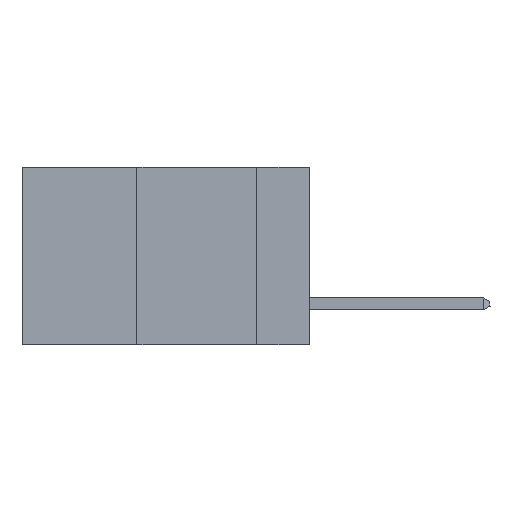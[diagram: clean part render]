
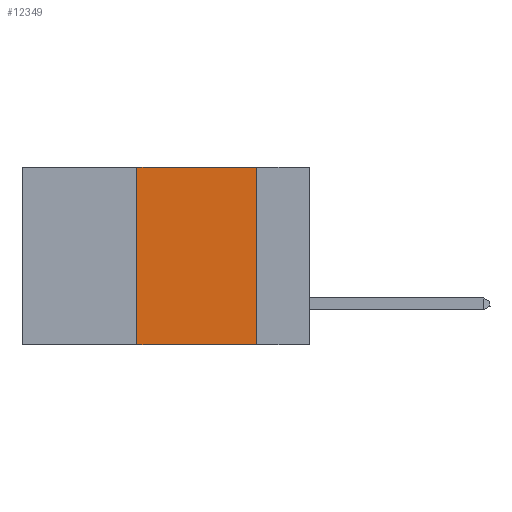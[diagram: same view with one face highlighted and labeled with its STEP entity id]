
A CAD part, left-side view. The second image highlights one B-rep face of the part: STEP entity #12349.
In plain terms, the highlighted planar face has unit normal (-1, 0, 0).
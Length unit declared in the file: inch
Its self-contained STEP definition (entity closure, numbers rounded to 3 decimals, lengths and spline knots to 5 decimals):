
#645 = DIRECTION ( 'NONE',  ( 0., -1., 0. ) ) ;
#769 = CARTESIAN_POINT ( 'NONE',  ( 0., 0.6, 0. ) ) ;
#1756 = AXIS2_PLACEMENT_3D ( 'NONE', #13225, #12347, #5356 ) ;
#1812 = LINE ( 'NONE', #769, #12494 ) ;
#2171 = DIRECTION ( 'NONE',  ( 0., 0., 1. ) ) ;
#2660 = EDGE_LOOP ( 'NONE', ( #5805, #11020, #7889, #4218 ) ) ;
#3350 = EDGE_CURVE ( 'NONE', #5940, #10086, #7661, .T. ) ;
#3627 = DIRECTION ( 'NONE',  ( 0., -1., 0. ) ) ;
#4139 = VECTOR ( 'NONE', #645, 39.37008 ) ;
#4218 = ORIENTED_EDGE ( 'NONE', *, *, #3350, .T. ) ;
#4320 = VERTEX_POINT ( 'NONE', #4525 ) ;
#4436 = VECTOR ( 'NONE', #2171, 39.37008 ) ;
#4525 = CARTESIAN_POINT ( 'NONE',  ( 0., 0.11, 0. ) ) ;
#4594 = LINE ( 'NONE', #12316, #4436 ) ;
#5085 = EDGE_CURVE ( 'NONE', #5940, #8189, #4594, .T. ) ;
#5356 = DIRECTION ( 'NONE',  ( 0., 0., -1. ) ) ;
#5622 = CARTESIAN_POINT ( 'NONE',  ( 0., 0.36, -0.37 ) ) ;
#5805 = ORIENTED_EDGE ( 'NONE', *, *, #8806, .F. ) ;
#5940 = VERTEX_POINT ( 'NONE', #5622 ) ;
#6126 = PLANE ( 'NONE',  #1756 ) ;
#6367 = CARTESIAN_POINT ( 'NONE',  ( 0., 0.36, 0. ) ) ;
#6561 = VECTOR ( 'NONE', #6746, 39.37008 ) ;
#6746 = DIRECTION ( 'NONE',  ( 0., 0., -1. ) ) ;
#7213 = EDGE_CURVE ( 'NONE', #8189, #4320, #1812, .T. ) ;
#7661 = LINE ( 'NONE', #7678, #4139 ) ;
#7678 = CARTESIAN_POINT ( 'NONE',  ( 0., 0.6, -0.37 ) ) ;
#7889 = ORIENTED_EDGE ( 'NONE', *, *, #5085, .F. ) ;
#8189 = VERTEX_POINT ( 'NONE', #6367 ) ;
#8553 = FACE_OUTER_BOUND ( 'NONE', #2660, .T. ) ;
#8806 = EDGE_CURVE ( 'NONE', #4320, #10086, #11028, .T. ) ;
#10086 = VERTEX_POINT ( 'NONE', #11660 ) ;
#11020 = ORIENTED_EDGE ( 'NONE', *, *, #7213, .F. ) ;
#11028 = LINE ( 'NONE', #12396, #6561 ) ;
#11660 = CARTESIAN_POINT ( 'NONE',  ( 0., 0.11, -0.37 ) ) ;
#12316 = CARTESIAN_POINT ( 'NONE',  ( 0., 0.36, 0. ) ) ;
#12347 = DIRECTION ( 'NONE',  ( 1., 0., 0. ) ) ;
#12349 = ADVANCED_FACE ( 'NONE', ( #8553 ), #6126, .F. ) ;
#12396 = CARTESIAN_POINT ( 'NONE',  ( 0., 0.11, 0. ) ) ;
#12494 = VECTOR ( 'NONE', #3627, 39.37008 ) ;
#13225 = CARTESIAN_POINT ( 'NONE',  ( 0., 0.6, 0. ) ) ;
